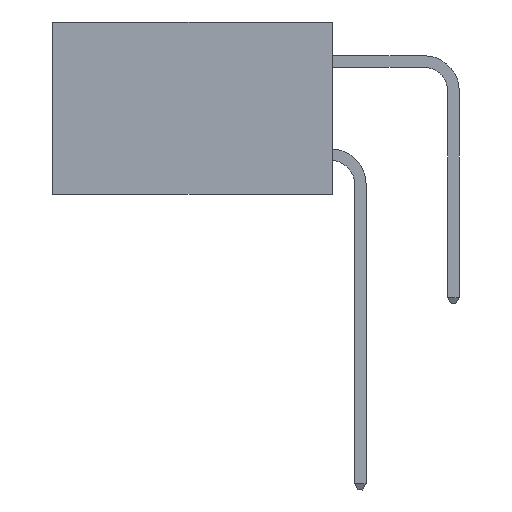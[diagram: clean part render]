
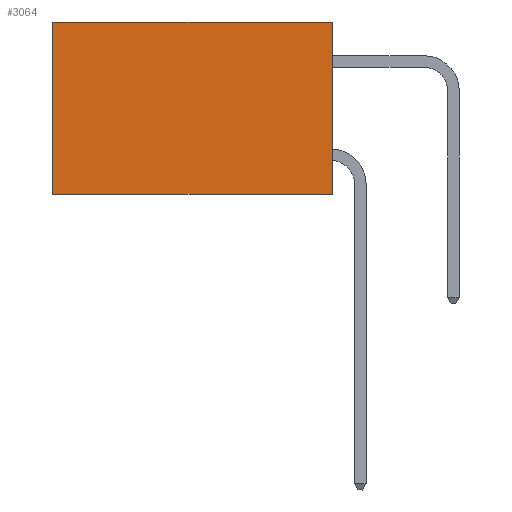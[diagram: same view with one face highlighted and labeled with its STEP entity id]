
A CAD part, left-side view. The second image highlights one B-rep face of the part: STEP entity #3064.
In plain terms, the highlighted planar face has unit normal (-1, 0, 0).
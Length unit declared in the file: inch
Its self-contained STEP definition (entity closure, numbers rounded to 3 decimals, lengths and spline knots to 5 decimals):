
#315 = DIRECTION ( 'NONE',  ( 0., 1., 0. ) ) ;
#650 = ORIENTED_EDGE ( 'NONE', *, *, #13004, .F. ) ;
#681 = ORIENTED_EDGE ( 'NONE', *, *, #8214, .F. ) ;
#796 = LINE ( 'NONE', #9129, #9636 ) ;
#1028 = CARTESIAN_POINT ( 'NONE',  ( 0.298, 0.6, -0.37 ) ) ;
#1705 = CARTESIAN_POINT ( 'NONE',  ( 0.298, 0., 0. ) ) ;
#1880 = DIRECTION ( 'NONE',  ( 1., 0., 0. ) ) ;
#2289 = VERTEX_POINT ( 'NONE', #13906 ) ;
#2916 = LINE ( 'NONE', #9315, #11958 ) ;
#2995 = VECTOR ( 'NONE', #10024, 39.37008 ) ;
#3064 = ADVANCED_FACE ( 'NONE', ( #8105 ), #14659, .F. ) ;
#6937 = CARTESIAN_POINT ( 'NONE',  ( 0.298, 0., 0. ) ) ;
#7559 = CARTESIAN_POINT ( 'NONE',  ( 0.298, 0., 0. ) ) ;
#7943 = DIRECTION ( 'NONE',  ( 0., 1., 0. ) ) ;
#8105 = FACE_OUTER_BOUND ( 'NONE', #12519, .T. ) ;
#8194 = DIRECTION ( 'NONE',  ( 0., 0., -1. ) ) ;
#8214 = EDGE_CURVE ( 'NONE', #9891, #2289, #8591, .T. ) ;
#8591 = LINE ( 'NONE', #12571, #2995 ) ;
#8726 = EDGE_CURVE ( 'NONE', #13744, #9006, #796, .T. ) ;
#9006 = VERTEX_POINT ( 'NONE', #1028 ) ;
#9129 = CARTESIAN_POINT ( 'NONE',  ( 0.298, 0.6, 0. ) ) ;
#9315 = CARTESIAN_POINT ( 'NONE',  ( 0.298, 0., -0.37 ) ) ;
#9636 = VECTOR ( 'NONE', #14286, 39.37008 ) ;
#9891 = VERTEX_POINT ( 'NONE', #7559 ) ;
#10024 = DIRECTION ( 'NONE',  ( 0., 0., -1. ) ) ;
#10108 = LINE ( 'NONE', #1705, #12335 ) ;
#11836 = CARTESIAN_POINT ( 'NONE',  ( 0.298, 0.6, 0. ) ) ;
#11958 = VECTOR ( 'NONE', #7943, 39.37008 ) ;
#12335 = VECTOR ( 'NONE', #315, 39.37008 ) ;
#12519 = EDGE_LOOP ( 'NONE', ( #12543, #650, #681, #16153 ) ) ;
#12543 = ORIENTED_EDGE ( 'NONE', *, *, #8726, .T. ) ;
#12571 = CARTESIAN_POINT ( 'NONE',  ( 0.298, 0., 0. ) ) ;
#12755 = AXIS2_PLACEMENT_3D ( 'NONE', #6937, #1880, #8194 ) ;
#13004 = EDGE_CURVE ( 'NONE', #2289, #9006, #2916, .T. ) ;
#13744 = VERTEX_POINT ( 'NONE', #11836 ) ;
#13782 = EDGE_CURVE ( 'NONE', #9891, #13744, #10108, .T. ) ;
#13906 = CARTESIAN_POINT ( 'NONE',  ( 0.298, 0., -0.37 ) ) ;
#14286 = DIRECTION ( 'NONE',  ( 0., 0., -1. ) ) ;
#14659 = PLANE ( 'NONE',  #12755 ) ;
#16153 = ORIENTED_EDGE ( 'NONE', *, *, #13782, .T. ) ;
